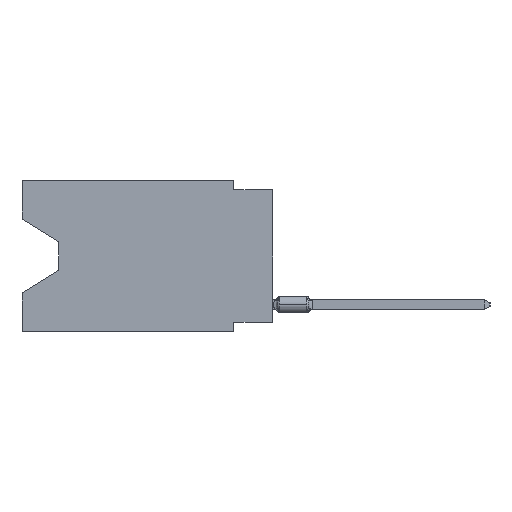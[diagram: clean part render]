
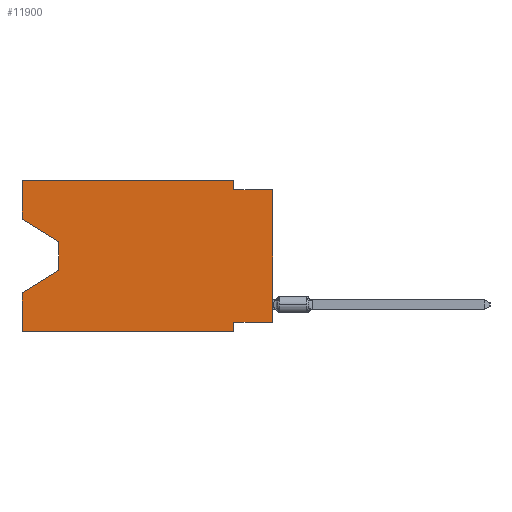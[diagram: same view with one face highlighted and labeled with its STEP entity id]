
A CAD part, left-side view. The second image highlights one B-rep face of the part: STEP entity #11900.
In plain terms, the highlighted planar face has unit normal (-1, 0, 0).
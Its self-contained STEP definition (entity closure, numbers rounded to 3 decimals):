
#441 = CARTESIAN_POINT ( 'NONE',  ( 0., 0., -9.271 ) ) ;
#3049 = CARTESIAN_POINT ( 'NONE',  ( 0., 16.383, 0. ) ) ;
#3081 = CARTESIAN_POINT ( 'NONE',  ( 0., 13.97, -4.013 ) ) ;
#4179 = CARTESIAN_POINT ( 'NONE',  ( 0., 16.383, 0. ) ) ;
#4319 = CARTESIAN_POINT ( 'NONE',  ( 0., 2.54, -9.906 ) ) ;
#4358 = ORIENTED_EDGE ( 'NONE', *, *, #77408, .T. ) ;
#4366 = CARTESIAN_POINT ( 'NONE',  ( 0., 16.383, 0. ) ) ;
#5696 = CARTESIAN_POINT ( 'NONE',  ( 0., 13.97, -5.893 ) ) ;
#6382 = VERTEX_POINT ( 'NONE', #80618 ) ;
#6507 = LINE ( 'NONE', #441, #12929 ) ;
#6576 = CARTESIAN_POINT ( 'NONE',  ( 0., 0., -0.635 ) ) ;
#7347 = CARTESIAN_POINT ( 'NONE',  ( 0., 13.97, -4.013 ) ) ;
#7495 = LINE ( 'NONE', #20026, #61749 ) ;
#9083 = VECTOR ( 'NONE', #64876, 1000. ) ;
#9177 = VERTEX_POINT ( 'NONE', #20492 ) ;
#9437 = LINE ( 'NONE', #30145, #83305 ) ;
#9673 = CARTESIAN_POINT ( 'NONE',  ( 0., 0., -9.271 ) ) ;
#11900 = ADVANCED_FACE ( 'NONE', ( #16540 ), #23442, .F. ) ;
#12145 = DIRECTION ( 'NONE',  ( 0., 0.855, -0.519 ) ) ;
#12626 = LINE ( 'NONE', #6576, #9083 ) ;
#12929 = VECTOR ( 'NONE', #46188, 1000. ) ;
#13961 = EDGE_CURVE ( 'NONE', #81430, #80294, #9437, .T. ) ;
#14247 = LINE ( 'NONE', #7347, #19903 ) ;
#15935 = CARTESIAN_POINT ( 'NONE',  ( 0., 2.54, -0.635 ) ) ;
#16289 = VECTOR ( 'NONE', #69946, 1000. ) ;
#16540 = FACE_OUTER_BOUND ( 'NONE', #36263, .T. ) ;
#16571 = ORIENTED_EDGE ( 'NONE', *, *, #33109, .T. ) ;
#17445 = EDGE_CURVE ( 'NONE', #75435, #6382, #12626, .T. ) ;
#17759 = VERTEX_POINT ( 'NONE', #76052 ) ;
#19829 = EDGE_CURVE ( 'NONE', #81430, #45629, #34670, .T. ) ;
#19903 = VECTOR ( 'NONE', #67772, 1000. ) ;
#20026 = CARTESIAN_POINT ( 'NONE',  ( 0., 16.383, -2.546 ) ) ;
#20492 = CARTESIAN_POINT ( 'NONE',  ( 0., 2.54, -9.271 ) ) ;
#22697 = CARTESIAN_POINT ( 'NONE',  ( 0., 2.54, 0. ) ) ;
#23001 = CARTESIAN_POINT ( 'NONE',  ( 0., 16.383, 0. ) ) ;
#23442 = PLANE ( 'NONE',  #30371 ) ;
#23761 = LINE ( 'NONE', #3049, #16289 ) ;
#24994 = CARTESIAN_POINT ( 'NONE',  ( 0., 2.54, 0. ) ) ;
#25061 = EDGE_CURVE ( 'NONE', #45647, #84476, #7495, .T. ) ;
#27188 = ORIENTED_EDGE ( 'NONE', *, *, #70680, .F. ) ;
#27360 = CARTESIAN_POINT ( 'NONE',  ( 0., 0., 0. ) ) ;
#28103 = CARTESIAN_POINT ( 'NONE',  ( 0., 16.383, -7.36 ) ) ;
#28184 = CARTESIAN_POINT ( 'NONE',  ( 0., 16.383, -9.906 ) ) ;
#28622 = DIRECTION ( 'NONE',  ( 0., -1., 0. ) ) ;
#29711 = VERTEX_POINT ( 'NONE', #22697 ) ;
#30145 = CARTESIAN_POINT ( 'NONE',  ( 0., 16.383, 0. ) ) ;
#30371 = AXIS2_PLACEMENT_3D ( 'NONE', #23001, #41975, #83009 ) ;
#33109 = EDGE_CURVE ( 'NONE', #62266, #6382, #53699, .T. ) ;
#34670 = LINE ( 'NONE', #28184, #75606 ) ;
#35400 = VECTOR ( 'NONE', #41319, 1000. ) ;
#36184 = ORIENTED_EDGE ( 'NONE', *, *, #73953, .F. ) ;
#36263 = EDGE_LOOP ( 'NONE', ( #64458, #69184, #4358, #58437, #54794, #36184, #45496, #16571, #66195, #70752, #57007, #27188 ) ) ;
#36328 = VECTOR ( 'NONE', #12145, 1000. ) ;
#41319 = DIRECTION ( 'NONE',  ( 0., 0., -1. ) ) ;
#41728 = CARTESIAN_POINT ( 'NONE',  ( 0., 2.54, -9.906 ) ) ;
#41975 = DIRECTION ( 'NONE',  ( 1., 0., 0. ) ) ;
#44472 = EDGE_CURVE ( 'NONE', #29711, #75435, #45683, .T. ) ;
#45496 = ORIENTED_EDGE ( 'NONE', *, *, #55596, .F. ) ;
#45629 = VERTEX_POINT ( 'NONE', #4319 ) ;
#45647 = VERTEX_POINT ( 'NONE', #82044 ) ;
#45683 = LINE ( 'NONE', #24994, #62887 ) ;
#46188 = DIRECTION ( 'NONE',  ( 0., 1., 0. ) ) ;
#53699 = LINE ( 'NONE', #27360, #82030 ) ;
#54527 = EDGE_CURVE ( 'NONE', #84476, #17759, #14247, .T. ) ;
#54794 = ORIENTED_EDGE ( 'NONE', *, *, #19829, .T. ) ;
#54832 = VECTOR ( 'NONE', #77314, 1000. ) ;
#55388 = DIRECTION ( 'NONE',  ( 0., 0., 1. ) ) ;
#55596 = EDGE_CURVE ( 'NONE', #62266, #9177, #6507, .T. ) ;
#57007 = ORIENTED_EDGE ( 'NONE', *, *, #75213, .F. ) ;
#58437 = ORIENTED_EDGE ( 'NONE', *, *, #13961, .F. ) ;
#60940 = CARTESIAN_POINT ( 'NONE',  ( 0., 16.383, -9.906 ) ) ;
#61749 = VECTOR ( 'NONE', #72707, 1000. ) ;
#62266 = VERTEX_POINT ( 'NONE', #9673 ) ;
#62887 = VECTOR ( 'NONE', #84156, 1000. ) ;
#64388 = LINE ( 'NONE', #5696, #36328 ) ;
#64458 = ORIENTED_EDGE ( 'NONE', *, *, #25061, .T. ) ;
#64876 = DIRECTION ( 'NONE',  ( 0., -1., 0. ) ) ;
#66195 = ORIENTED_EDGE ( 'NONE', *, *, #17445, .F. ) ;
#67772 = DIRECTION ( 'NONE',  ( 0., 0., -1. ) ) ;
#69184 = ORIENTED_EDGE ( 'NONE', *, *, #54527, .T. ) ;
#69853 = DIRECTION ( 'NONE',  ( 0., 0., 1. ) ) ;
#69946 = DIRECTION ( 'NONE',  ( 0., 0., 1. ) ) ;
#70680 = EDGE_CURVE ( 'NONE', #45647, #74116, #23761, .T. ) ;
#70752 = ORIENTED_EDGE ( 'NONE', *, *, #44472, .F. ) ;
#72707 = DIRECTION ( 'NONE',  ( 0., -0.855, -0.519 ) ) ;
#73953 = EDGE_CURVE ( 'NONE', #9177, #45629, #82769, .T. ) ;
#74116 = VERTEX_POINT ( 'NONE', #4179 ) ;
#75213 = EDGE_CURVE ( 'NONE', #74116, #29711, #76058, .T. ) ;
#75435 = VERTEX_POINT ( 'NONE', #15935 ) ;
#75606 = VECTOR ( 'NONE', #28622, 1000. ) ;
#76052 = CARTESIAN_POINT ( 'NONE',  ( 0., 13.97, -5.893 ) ) ;
#76058 = LINE ( 'NONE', #4366, #54832 ) ;
#77314 = DIRECTION ( 'NONE',  ( 0., -1., 0. ) ) ;
#77408 = EDGE_CURVE ( 'NONE', #17759, #80294, #64388, .T. ) ;
#80294 = VERTEX_POINT ( 'NONE', #28103 ) ;
#80618 = CARTESIAN_POINT ( 'NONE',  ( 0., 0., -0.635 ) ) ;
#81430 = VERTEX_POINT ( 'NONE', #60940 ) ;
#82030 = VECTOR ( 'NONE', #55388, 1000. ) ;
#82044 = CARTESIAN_POINT ( 'NONE',  ( 0., 16.383, -2.546 ) ) ;
#82769 = LINE ( 'NONE', #41728, #35400 ) ;
#83009 = DIRECTION ( 'NONE',  ( 0., 0., -1. ) ) ;
#83305 = VECTOR ( 'NONE', #69853, 1000. ) ;
#84156 = DIRECTION ( 'NONE',  ( 0., 0., -1. ) ) ;
#84476 = VERTEX_POINT ( 'NONE', #3081 ) ;
